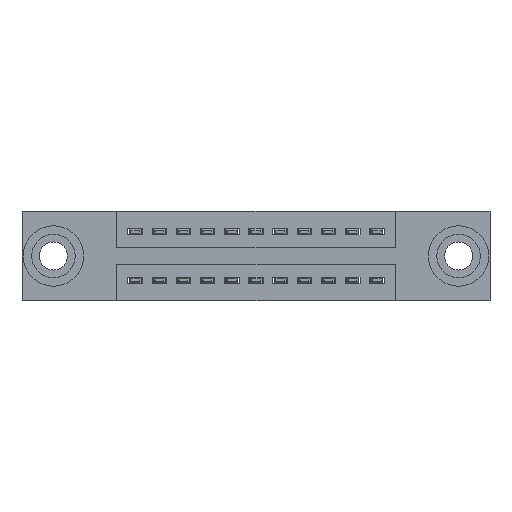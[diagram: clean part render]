
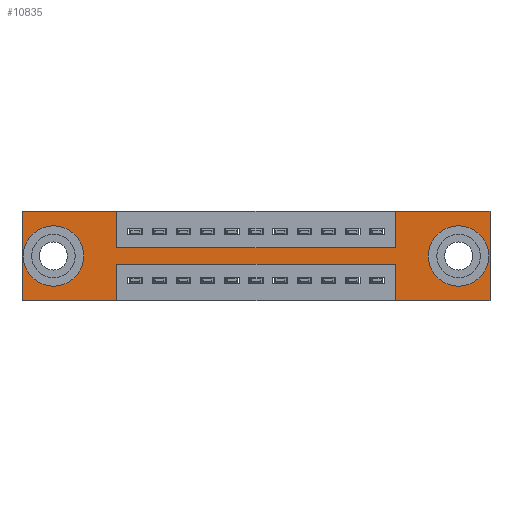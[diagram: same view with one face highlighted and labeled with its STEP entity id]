
A CAD part, front view. The second image highlights one B-rep face of the part: STEP entity #10835.
In plain terms, the highlighted planar face has unit normal (0, -1, 0).
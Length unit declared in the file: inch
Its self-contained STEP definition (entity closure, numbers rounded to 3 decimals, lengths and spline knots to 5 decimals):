
#17 = VERTEX_POINT ( 'NONE', #4257 ) ;
#291 = PLANE ( 'NONE',  #5717 ) ;
#465 = DIRECTION ( 'NONE',  ( 0., 1., 0. ) ) ;
#484 = ORIENTED_EDGE ( 'NONE', *, *, #8345, .F. ) ;
#535 = VECTOR ( 'NONE', #4365, 39.37008 ) ;
#743 = EDGE_LOOP ( 'NONE', ( #5215, #11304 ) ) ;
#903 = VERTEX_POINT ( 'NONE', #9301 ) ;
#943 = LINE ( 'NONE', #12464, #13131 ) ;
#1029 = EDGE_CURVE ( 'NONE', #6508, #17, #12316, .T. ) ;
#1110 = EDGE_LOOP ( 'NONE', ( #3016, #12624, #9493, #7036, #9612, #9809, #6829, #484, #6126, #12765, #4580, #5171 ) ) ;
#1117 = VERTEX_POINT ( 'NONE', #1745 ) ;
#1181 = EDGE_CURVE ( 'NONE', #1514, #4892, #8296, .T. ) ;
#1203 = CARTESIAN_POINT ( 'NONE',  ( 0., 0., 0. ) ) ;
#1313 = VECTOR ( 'NONE', #3342, 39.37008 ) ;
#1322 = DIRECTION ( 'NONE',  ( -1., 0., 0. ) ) ;
#1353 = EDGE_CURVE ( 'NONE', #7782, #3241, #4307, .T. ) ;
#1436 = VECTOR ( 'NONE', #1528, 39.37008 ) ;
#1449 = DIRECTION ( 'NONE',  ( 0., 0., -1. ) ) ;
#1467 = CARTESIAN_POINT ( 'NONE',  ( 0., 0., -0.37 ) ) ;
#1514 = VERTEX_POINT ( 'NONE', #13226 ) ;
#1528 = DIRECTION ( 'NONE',  ( 1., 0., 0. ) ) ;
#1745 = CARTESIAN_POINT ( 'NONE',  ( 1.5425, 0., 0. ) ) ;
#1835 = EDGE_CURVE ( 'NONE', #11487, #1514, #943, .T. ) ;
#2222 = CARTESIAN_POINT ( 'NONE',  ( 0.3925, 0., -0.22 ) ) ;
#2403 = LINE ( 'NONE', #2222, #7322 ) ;
#2612 = CARTESIAN_POINT ( 'NONE',  ( 1.935, 0., 0. ) ) ;
#2844 = LINE ( 'NONE', #1467, #12772 ) ;
#3016 = ORIENTED_EDGE ( 'NONE', *, *, #1835, .F. ) ;
#3216 = EDGE_CURVE ( 'NONE', #4772, #10588, #10762, .T. ) ;
#3241 = VERTEX_POINT ( 'NONE', #10459 ) ;
#3272 = DIRECTION ( 'NONE',  ( 0., 1., 0. ) ) ;
#3302 = CARTESIAN_POINT ( 'NONE',  ( 1.5425, 0., -0.37 ) ) ;
#3342 = DIRECTION ( 'NONE',  ( 0., 0., 1. ) ) ;
#3366 = DIRECTION ( 'NONE',  ( 0., 0., 1. ) ) ;
#3542 = CARTESIAN_POINT ( 'NONE',  ( 0., 0., 0. ) ) ;
#3643 = VERTEX_POINT ( 'NONE', #9356 ) ;
#3775 = DIRECTION ( 'NONE',  ( 0., 1., 0. ) ) ;
#3838 = VECTOR ( 'NONE', #4955, 39.37008 ) ;
#4070 = VECTOR ( 'NONE', #7762, 39.37008 ) ;
#4122 = VERTEX_POINT ( 'NONE', #1203 ) ;
#4257 = CARTESIAN_POINT ( 'NONE',  ( 1.805, 0., -0.263 ) ) ;
#4281 = CARTESIAN_POINT ( 'NONE',  ( 1.805, 0., -0.185 ) ) ;
#4307 = LINE ( 'NONE', #2612, #11512 ) ;
#4365 = DIRECTION ( 'NONE',  ( 1., 0., 0. ) ) ;
#4434 = DIRECTION ( 'NONE',  ( 0., 0., 1. ) ) ;
#4500 = CARTESIAN_POINT ( 'NONE',  ( 0.3925, 0., -0.15 ) ) ;
#4524 = CARTESIAN_POINT ( 'NONE',  ( 0., 0., 0. ) ) ;
#4580 = ORIENTED_EDGE ( 'NONE', *, *, #12669, .F. ) ;
#4594 = CARTESIAN_POINT ( 'NONE',  ( 0.3925, 0., 0. ) ) ;
#4697 = EDGE_LOOP ( 'NONE', ( #8429, #12120 ) ) ;
#4772 = VERTEX_POINT ( 'NONE', #3302 ) ;
#4872 = CARTESIAN_POINT ( 'NONE',  ( 1.805, 0., -0.107 ) ) ;
#4892 = VERTEX_POINT ( 'NONE', #8567 ) ;
#4955 = DIRECTION ( 'NONE',  ( -1., 0., 0. ) ) ;
#5030 = VECTOR ( 'NONE', #4434, 39.37008 ) ;
#5137 = AXIS2_PLACEMENT_3D ( 'NONE', #8481, #3272, #5429 ) ;
#5171 = ORIENTED_EDGE ( 'NONE', *, *, #1181, .F. ) ;
#5215 = ORIENTED_EDGE ( 'NONE', *, *, #12560, .T. ) ;
#5221 = CIRCLE ( 'NONE', #12769, 0.078 ) ;
#5243 = CARTESIAN_POINT ( 'NONE',  ( 1.935, 0., 0. ) ) ;
#5429 = DIRECTION ( 'NONE',  ( 0., 0., 1. ) ) ;
#5717 = AXIS2_PLACEMENT_3D ( 'NONE', #8425, #9425, #7336 ) ;
#5929 = AXIS2_PLACEMENT_3D ( 'NONE', #8950, #3775, #10915 ) ;
#6126 = ORIENTED_EDGE ( 'NONE', *, *, #7406, .F. ) ;
#6209 = EDGE_CURVE ( 'NONE', #3241, #4772, #2844, .T. ) ;
#6224 = DIRECTION ( 'NONE',  ( 0., 1., 0. ) ) ;
#6250 = DIRECTION ( 'NONE',  ( 0., 0., -1. ) ) ;
#6423 = VERTEX_POINT ( 'NONE', #9983 ) ;
#6508 = VERTEX_POINT ( 'NONE', #4872 ) ;
#6675 = FACE_OUTER_BOUND ( 'NONE', #1110, .T. ) ;
#6720 = EDGE_CURVE ( 'NONE', #11750, #1117, #10202, .T. ) ;
#6829 = ORIENTED_EDGE ( 'NONE', *, *, #6720, .F. ) ;
#7036 = ORIENTED_EDGE ( 'NONE', *, *, #6209, .F. ) ;
#7322 = VECTOR ( 'NONE', #1322, 39.37008 ) ;
#7336 = DIRECTION ( 'NONE',  ( 0., 0., -1. ) ) ;
#7406 = EDGE_CURVE ( 'NONE', #7827, #3643, #12409, .T. ) ;
#7739 = CIRCLE ( 'NONE', #5137, 0.078 ) ;
#7762 = DIRECTION ( 'NONE',  ( 1., 0., 0. ) ) ;
#7782 = VERTEX_POINT ( 'NONE', #5243 ) ;
#7827 = VERTEX_POINT ( 'NONE', #13051 ) ;
#8011 = EDGE_CURVE ( 'NONE', #4122, #7827, #9989, .T. ) ;
#8012 = EDGE_CURVE ( 'NONE', #903, #6423, #13216, .T. ) ;
#8204 = AXIS2_PLACEMENT_3D ( 'NONE', #4281, #465, #9559 ) ;
#8296 = LINE ( 'NONE', #10999, #3838 ) ;
#8345 = EDGE_CURVE ( 'NONE', #3643, #11750, #8870, .T. ) ;
#8392 = LINE ( 'NONE', #4524, #5030 ) ;
#8425 = CARTESIAN_POINT ( 'NONE',  ( 0., 0., -0.37 ) ) ;
#8429 = ORIENTED_EDGE ( 'NONE', *, *, #1029, .T. ) ;
#8480 = CARTESIAN_POINT ( 'NONE',  ( 1.5425, 0., -0.22 ) ) ;
#8481 = CARTESIAN_POINT ( 'NONE',  ( 0.13, 0., -0.185 ) ) ;
#8567 = CARTESIAN_POINT ( 'NONE',  ( 0., 0., -0.37 ) ) ;
#8870 = LINE ( 'NONE', #4500, #535 ) ;
#8873 = DIRECTION ( 'NONE',  ( 0., 0., -1. ) ) ;
#8950 = CARTESIAN_POINT ( 'NONE',  ( 0.13, 0., -0.185 ) ) ;
#9085 = VECTOR ( 'NONE', #3366, 39.37008 ) ;
#9255 = FACE_BOUND ( 'NONE', #4697, .T. ) ;
#9301 = CARTESIAN_POINT ( 'NONE',  ( 0.13, 0., -0.263 ) ) ;
#9356 = CARTESIAN_POINT ( 'NONE',  ( 0.3925, 0., -0.15 ) ) ;
#9425 = DIRECTION ( 'NONE',  ( 0., -1., 0. ) ) ;
#9493 = ORIENTED_EDGE ( 'NONE', *, *, #3216, .F. ) ;
#9559 = DIRECTION ( 'NONE',  ( 0., 0., -1. ) ) ;
#9612 = ORIENTED_EDGE ( 'NONE', *, *, #1353, .F. ) ;
#9686 = VECTOR ( 'NONE', #11755, 39.37008 ) ;
#9788 = CARTESIAN_POINT ( 'NONE',  ( 0., 0., 0. ) ) ;
#9809 = ORIENTED_EDGE ( 'NONE', *, *, #10342, .F. ) ;
#9881 = FACE_BOUND ( 'NONE', #743, .T. ) ;
#9983 = CARTESIAN_POINT ( 'NONE',  ( 0.13, 0., -0.107 ) ) ;
#9989 = LINE ( 'NONE', #9788, #4070 ) ;
#9990 = EDGE_CURVE ( 'NONE', #10588, #11487, #2403, .T. ) ;
#10202 = LINE ( 'NONE', #12566, #9085 ) ;
#10342 = EDGE_CURVE ( 'NONE', #1117, #7782, #11021, .T. ) ;
#10459 = CARTESIAN_POINT ( 'NONE',  ( 1.935, 0., -0.37 ) ) ;
#10547 = CARTESIAN_POINT ( 'NONE',  ( 1.5425, 0., -0.37 ) ) ;
#10588 = VERTEX_POINT ( 'NONE', #8480 ) ;
#10631 = CARTESIAN_POINT ( 'NONE',  ( 0.3925, 0., -0.22 ) ) ;
#10762 = LINE ( 'NONE', #10547, #1313 ) ;
#10835 = ADVANCED_FACE ( 'NONE', ( #9255, #9881, #6675 ), #291, .T. ) ;
#10915 = DIRECTION ( 'NONE',  ( 0., 0., 1. ) ) ;
#10999 = CARTESIAN_POINT ( 'NONE',  ( 0., 0., -0.37 ) ) ;
#11021 = LINE ( 'NONE', #3542, #1436 ) ;
#11137 = CARTESIAN_POINT ( 'NONE',  ( 1.5425, 0., -0.15 ) ) ;
#11304 = ORIENTED_EDGE ( 'NONE', *, *, #8012, .T. ) ;
#11487 = VERTEX_POINT ( 'NONE', #10631 ) ;
#11512 = VECTOR ( 'NONE', #8873, 39.37008 ) ;
#11609 = DIRECTION ( 'NONE',  ( -1., 0., 0. ) ) ;
#11616 = EDGE_CURVE ( 'NONE', #17, #6508, #5221, .T. ) ;
#11750 = VERTEX_POINT ( 'NONE', #11137 ) ;
#11755 = DIRECTION ( 'NONE',  ( 0., 0., -1. ) ) ;
#12120 = ORIENTED_EDGE ( 'NONE', *, *, #11616, .T. ) ;
#12316 = CIRCLE ( 'NONE', #8204, 0.078 ) ;
#12394 = CARTESIAN_POINT ( 'NONE',  ( 1.805, 0., -0.185 ) ) ;
#12409 = LINE ( 'NONE', #4594, #9686 ) ;
#12464 = CARTESIAN_POINT ( 'NONE',  ( 0.3925, 0., -0.37 ) ) ;
#12560 = EDGE_CURVE ( 'NONE', #6423, #903, #7739, .T. ) ;
#12566 = CARTESIAN_POINT ( 'NONE',  ( 1.5425, 0., 0. ) ) ;
#12624 = ORIENTED_EDGE ( 'NONE', *, *, #9990, .F. ) ;
#12669 = EDGE_CURVE ( 'NONE', #4892, #4122, #8392, .T. ) ;
#12765 = ORIENTED_EDGE ( 'NONE', *, *, #8011, .F. ) ;
#12769 = AXIS2_PLACEMENT_3D ( 'NONE', #12394, #6224, #1449 ) ;
#12772 = VECTOR ( 'NONE', #11609, 39.37008 ) ;
#13051 = CARTESIAN_POINT ( 'NONE',  ( 0.3925, 0., 0. ) ) ;
#13131 = VECTOR ( 'NONE', #6250, 39.37008 ) ;
#13216 = CIRCLE ( 'NONE', #5929, 0.078 ) ;
#13226 = CARTESIAN_POINT ( 'NONE',  ( 0.3925, 0., -0.37 ) ) ;
